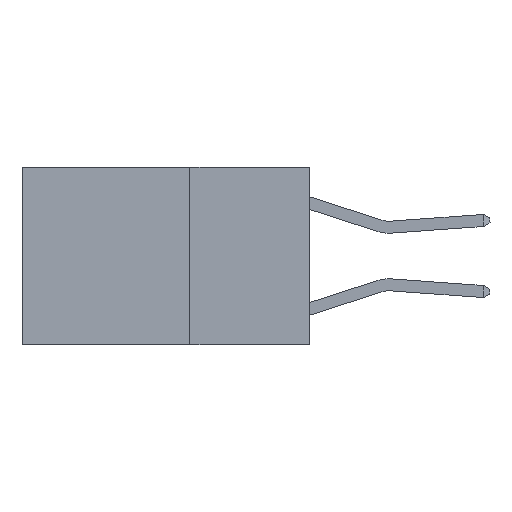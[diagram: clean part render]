
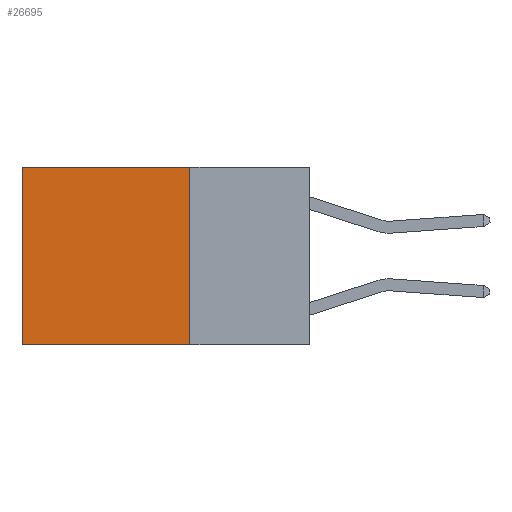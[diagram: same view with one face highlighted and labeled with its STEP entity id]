
A CAD part, left-side view. The second image highlights one B-rep face of the part: STEP entity #26695.
In plain terms, the highlighted planar face has unit normal (-1, 0, 0).
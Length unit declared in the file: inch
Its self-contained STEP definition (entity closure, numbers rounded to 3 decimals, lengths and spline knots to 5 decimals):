
#1563 = LINE ( 'NONE', #22108, #24918 ) ;
#1652 = VECTOR ( 'NONE', #17330, 39.37008 ) ;
#1986 = EDGE_LOOP ( 'NONE', ( #30067, #25102, #21079, #11909 ) ) ;
#2589 = DIRECTION ( 'NONE',  ( 0., 0., -1. ) ) ;
#3123 = VERTEX_POINT ( 'NONE', #7667 ) ;
#3315 = EDGE_CURVE ( 'NONE', #3123, #23373, #6814, .T. ) ;
#6814 = LINE ( 'NONE', #15432, #18551 ) ;
#7667 = CARTESIAN_POINT ( 'NONE',  ( 0.2625, 0.25, -0.37 ) ) ;
#7718 = LINE ( 'NONE', #16583, #26319 ) ;
#8210 = VERTEX_POINT ( 'NONE', #19075 ) ;
#8365 = EDGE_CURVE ( 'NONE', #10380, #3123, #20322, .T. ) ;
#9709 = FACE_OUTER_BOUND ( 'NONE', #1986, .T. ) ;
#9793 = EDGE_CURVE ( 'NONE', #10380, #8210, #1563, .T. ) ;
#10380 = VERTEX_POINT ( 'NONE', #22195 ) ;
#10691 = EDGE_CURVE ( 'NONE', #8210, #23373, #7718, .T. ) ;
#11770 = CARTESIAN_POINT ( 'NONE',  ( 0.2625, 0.25, 0. ) ) ;
#11909 = ORIENTED_EDGE ( 'NONE', *, *, #9793, .T. ) ;
#14125 = DIRECTION ( 'NONE',  ( 0., 0., -1. ) ) ;
#15182 = DIRECTION ( 'NONE',  ( 0., 1., 0. ) ) ;
#15432 = CARTESIAN_POINT ( 'NONE',  ( 0.2625, 0.25, -0.37 ) ) ;
#16583 = CARTESIAN_POINT ( 'NONE',  ( 0.2625, 0.6, 0. ) ) ;
#17330 = DIRECTION ( 'NONE',  ( 0., 0., -1. ) ) ;
#18249 = AXIS2_PLACEMENT_3D ( 'NONE', #11770, #28056, #14125 ) ;
#18551 = VECTOR ( 'NONE', #27005, 39.37008 ) ;
#18747 = PLANE ( 'NONE',  #18249 ) ;
#19075 = CARTESIAN_POINT ( 'NONE',  ( 0.2625, 0.6, 0. ) ) ;
#20322 = LINE ( 'NONE', #28856, #1652 ) ;
#21079 = ORIENTED_EDGE ( 'NONE', *, *, #8365, .F. ) ;
#22108 = CARTESIAN_POINT ( 'NONE',  ( 0.2625, 0.25, 0. ) ) ;
#22195 = CARTESIAN_POINT ( 'NONE',  ( 0.2625, 0.25, 0. ) ) ;
#23373 = VERTEX_POINT ( 'NONE', #26160 ) ;
#24918 = VECTOR ( 'NONE', #15182, 39.37008 ) ;
#25102 = ORIENTED_EDGE ( 'NONE', *, *, #3315, .F. ) ;
#26160 = CARTESIAN_POINT ( 'NONE',  ( 0.2625, 0.6, -0.37 ) ) ;
#26319 = VECTOR ( 'NONE', #2589, 39.37008 ) ;
#26695 = ADVANCED_FACE ( 'NONE', ( #9709 ), #18747, .F. ) ;
#27005 = DIRECTION ( 'NONE',  ( 0., 1., 0. ) ) ;
#28056 = DIRECTION ( 'NONE',  ( 1., 0., 0. ) ) ;
#28856 = CARTESIAN_POINT ( 'NONE',  ( 0.2625, 0.25, 0. ) ) ;
#30067 = ORIENTED_EDGE ( 'NONE', *, *, #10691, .T. ) ;
